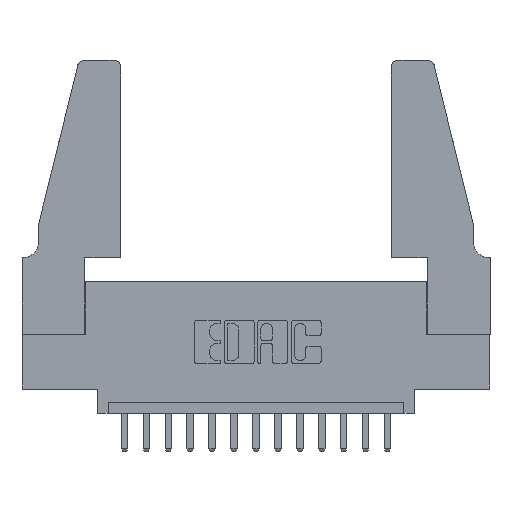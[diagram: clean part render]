
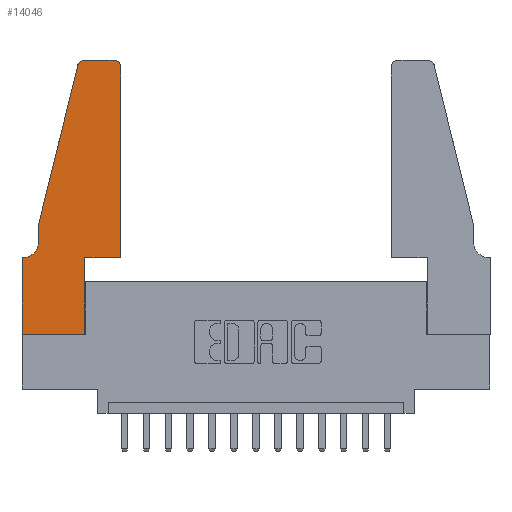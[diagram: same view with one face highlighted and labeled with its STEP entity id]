
A CAD part, top view. The second image highlights one B-rep face of the part: STEP entity #14046.
In plain terms, the highlighted planar face has unit normal (0, 0, 1).
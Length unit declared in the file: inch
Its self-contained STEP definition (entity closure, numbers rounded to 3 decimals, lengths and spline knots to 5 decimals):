
#88 = CARTESIAN_POINT ( 'NONE',  ( 0.0755, 0.35, 0.37 ) ) ;
#135 = EDGE_CURVE ( 'NONE', #14213, #14038, #9366, .T. ) ;
#304 = CARTESIAN_POINT ( 'NONE',  ( 0.4205, 1.25, 0.37 ) ) ;
#438 = EDGE_LOOP ( 'NONE', ( #8018, #10160, #13026, #11391, #10543, #615, #8445, #14098, #15376, #10660, #14527, #13093 ) ) ;
#490 = CARTESIAN_POINT ( 'NONE',  ( 0.4505, 1.22, 0.37 ) ) ;
#615 = ORIENTED_EDGE ( 'NONE', *, *, #1626, .T. ) ;
#939 = VERTEX_POINT ( 'NONE', #8569 ) ;
#1083 = CARTESIAN_POINT ( 'NONE',  ( 0.0055, 0.42, 0.37 ) ) ;
#1404 = CARTESIAN_POINT ( 'NONE',  ( 0.4205, 1.22, 0.37 ) ) ;
#1626 = EDGE_CURVE ( 'NONE', #5501, #11760, #2868, .T. ) ;
#1654 = VECTOR ( 'NONE', #7243, 39.37008 ) ;
#1736 = EDGE_CURVE ( 'NONE', #2744, #5074, #10662, .T. ) ;
#1775 = VERTEX_POINT ( 'NONE', #304 ) ;
#2022 = FACE_OUTER_BOUND ( 'NONE', #438, .T. ) ;
#2072 = EDGE_CURVE ( 'NONE', #1775, #14213, #10826, .T. ) ;
#2248 = CARTESIAN_POINT ( 'NONE',  ( 0., 0., 0.37 ) ) ;
#2744 = VERTEX_POINT ( 'NONE', #5267 ) ;
#2868 = LINE ( 'NONE', #88, #9099 ) ;
#2877 = CARTESIAN_POINT ( 'NONE',  ( 0.0755, 0.42, 0.37 ) ) ;
#2886 = DIRECTION ( 'NONE',  ( -1., 0., 0. ) ) ;
#3111 = LINE ( 'NONE', #5768, #9172 ) ;
#3594 = VERTEX_POINT ( 'NONE', #7405 ) ;
#3616 = CARTESIAN_POINT ( 'NONE',  ( 0., 0., 0.37 ) ) ;
#3851 = VERTEX_POINT ( 'NONE', #2248 ) ;
#4310 = CARTESIAN_POINT ( 'NONE',  ( 0.0755, 0.5, 0.37 ) ) ;
#4491 = VECTOR ( 'NONE', #10141, 39.37008 ) ;
#4787 = DIRECTION ( 'NONE',  ( 0., -1., 0. ) ) ;
#4941 = AXIS2_PLACEMENT_3D ( 'NONE', #15183, #6441, #11245 ) ;
#5074 = VERTEX_POINT ( 'NONE', #490 ) ;
#5188 = VECTOR ( 'NONE', #15541, 39.37008 ) ;
#5259 = CARTESIAN_POINT ( 'NONE',  ( 0.4505, 0.35, 0.37 ) ) ;
#5267 = CARTESIAN_POINT ( 'NONE',  ( 0.4505, 0.35, 0.37 ) ) ;
#5394 = CIRCLE ( 'NONE', #10179, 0.03 ) ;
#5398 = AXIS2_PLACEMENT_3D ( 'NONE', #9621, #8361, #7245 ) ;
#5501 = VERTEX_POINT ( 'NONE', #15202 ) ;
#5556 = VERTEX_POINT ( 'NONE', #2877 ) ;
#5668 = LINE ( 'NONE', #3616, #8625 ) ;
#5768 = CARTESIAN_POINT ( 'NONE',  ( 0.2865, 0.35, 0.37 ) ) ;
#5887 = LINE ( 'NONE', #6003, #1654 ) ;
#6003 = CARTESIAN_POINT ( 'NONE',  ( 0.4505, 0.35, 0.37 ) ) ;
#6166 = CARTESIAN_POINT ( 'NONE',  ( 0.0755, 0.5, 0.37 ) ) ;
#6428 = EDGE_CURVE ( 'NONE', #8971, #5556, #7143, .T. ) ;
#6441 = DIRECTION ( 'NONE',  ( 0., 0., 1. ) ) ;
#6452 = CARTESIAN_POINT ( 'NONE',  ( 0.0755, 0.5, 0.37 ) ) ;
#6761 = DIRECTION ( 'NONE',  ( 0., -1., 0. ) ) ;
#6926 = VECTOR ( 'NONE', #11486, 39.37008 ) ;
#7143 = LINE ( 'NONE', #6452, #9332 ) ;
#7243 = DIRECTION ( 'NONE',  ( 1., 0., 0. ) ) ;
#7245 = DIRECTION ( 'NONE',  ( 1., 0., 0. ) ) ;
#7405 = CARTESIAN_POINT ( 'NONE',  ( 0.2865, 0.35, 0.37 ) ) ;
#7954 = EDGE_CURVE ( 'NONE', #5074, #1775, #5394, .T. ) ;
#8018 = ORIENTED_EDGE ( 'NONE', *, *, #2072, .T. ) ;
#8102 = VECTOR ( 'NONE', #14927, 39.37008 ) ;
#8209 = DIRECTION ( 'NONE',  ( 0., 0., -1. ) ) ;
#8361 = DIRECTION ( 'NONE',  ( 0., 0., 1. ) ) ;
#8437 = EDGE_CURVE ( 'NONE', #14038, #8971, #9476, .T. ) ;
#8445 = ORIENTED_EDGE ( 'NONE', *, *, #11779, .T. ) ;
#8569 = CARTESIAN_POINT ( 'NONE',  ( 0.2865, 0., 0.37 ) ) ;
#8625 = VECTOR ( 'NONE', #4787, 39.37008 ) ;
#8760 = CARTESIAN_POINT ( 'NONE',  ( 0.25487, 1.22718, 0.37 ) ) ;
#8971 = VERTEX_POINT ( 'NONE', #6166 ) ;
#9099 = VECTOR ( 'NONE', #10993, 39.37008 ) ;
#9172 = VECTOR ( 'NONE', #13312, 39.37008 ) ;
#9254 = CIRCLE ( 'NONE', #9934, 0.07 ) ;
#9332 = VECTOR ( 'NONE', #6761, 39.37008 ) ;
#9366 = CIRCLE ( 'NONE', #5398, 0.03 ) ;
#9476 = LINE ( 'NONE', #4310, #5188 ) ;
#9621 = CARTESIAN_POINT ( 'NONE',  ( 0.284, 1.22, 0.37 ) ) ;
#9934 = AXIS2_PLACEMENT_3D ( 'NONE', #1083, #8209, #2886 ) ;
#10141 = DIRECTION ( 'NONE',  ( 1., 0., 0. ) ) ;
#10160 = ORIENTED_EDGE ( 'NONE', *, *, #135, .T. ) ;
#10179 = AXIS2_PLACEMENT_3D ( 'NONE', #1404, #13918, #15167 ) ;
#10543 = ORIENTED_EDGE ( 'NONE', *, *, #10697, .T. ) ;
#10660 = ORIENTED_EDGE ( 'NONE', *, *, #14006, .T. ) ;
#10662 = LINE ( 'NONE', #5259, #6926 ) ;
#10697 = EDGE_CURVE ( 'NONE', #5556, #5501, #9254, .T. ) ;
#10826 = LINE ( 'NONE', #14780, #8102 ) ;
#10993 = DIRECTION ( 'NONE',  ( -1., 0., 0. ) ) ;
#11245 = DIRECTION ( 'NONE',  ( 1., 0., 0. ) ) ;
#11391 = ORIENTED_EDGE ( 'NONE', *, *, #6428, .T. ) ;
#11486 = DIRECTION ( 'NONE',  ( 0., 1., 0. ) ) ;
#11760 = VERTEX_POINT ( 'NONE', #12315 ) ;
#11779 = EDGE_CURVE ( 'NONE', #11760, #3851, #5668, .T. ) ;
#12315 = CARTESIAN_POINT ( 'NONE',  ( 0., 0.35, 0.37 ) ) ;
#13026 = ORIENTED_EDGE ( 'NONE', *, *, #8437, .T. ) ;
#13093 = ORIENTED_EDGE ( 'NONE', *, *, #7954, .T. ) ;
#13312 = DIRECTION ( 'NONE',  ( 0., 1., 0. ) ) ;
#13918 = DIRECTION ( 'NONE',  ( 0., 0., 1. ) ) ;
#14006 = EDGE_CURVE ( 'NONE', #3594, #2744, #5887, .T. ) ;
#14012 = CARTESIAN_POINT ( 'NONE',  ( 0., 0., 0.37 ) ) ;
#14038 = VERTEX_POINT ( 'NONE', #8760 ) ;
#14046 = ADVANCED_FACE ( 'NONE', ( #2022 ), #15078, .T. ) ;
#14098 = ORIENTED_EDGE ( 'NONE', *, *, #15216, .T. ) ;
#14213 = VERTEX_POINT ( 'NONE', #14458 ) ;
#14458 = CARTESIAN_POINT ( 'NONE',  ( 0.284, 1.25, 0.37 ) ) ;
#14527 = ORIENTED_EDGE ( 'NONE', *, *, #1736, .T. ) ;
#14780 = CARTESIAN_POINT ( 'NONE',  ( 0.2605, 1.25, 0.37 ) ) ;
#14927 = DIRECTION ( 'NONE',  ( -1., 0., 0. ) ) ;
#15078 = PLANE ( 'NONE',  #4941 ) ;
#15167 = DIRECTION ( 'NONE',  ( 1., 0., 0. ) ) ;
#15183 = CARTESIAN_POINT ( 'NONE',  ( 0., 0.35, 0.37 ) ) ;
#15202 = CARTESIAN_POINT ( 'NONE',  ( 0.0055, 0.35, 0.37 ) ) ;
#15216 = EDGE_CURVE ( 'NONE', #3851, #939, #15432, .T. ) ;
#15376 = ORIENTED_EDGE ( 'NONE', *, *, #15894, .T. ) ;
#15432 = LINE ( 'NONE', #14012, #4491 ) ;
#15541 = DIRECTION ( 'NONE',  ( -0.239, -0.971, 0. ) ) ;
#15894 = EDGE_CURVE ( 'NONE', #939, #3594, #3111, .T. ) ;
